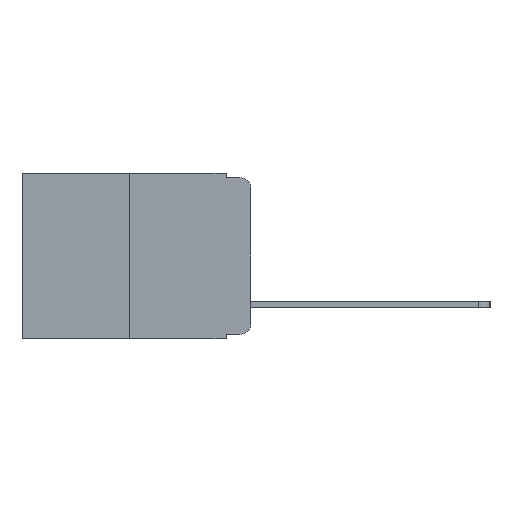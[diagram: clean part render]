
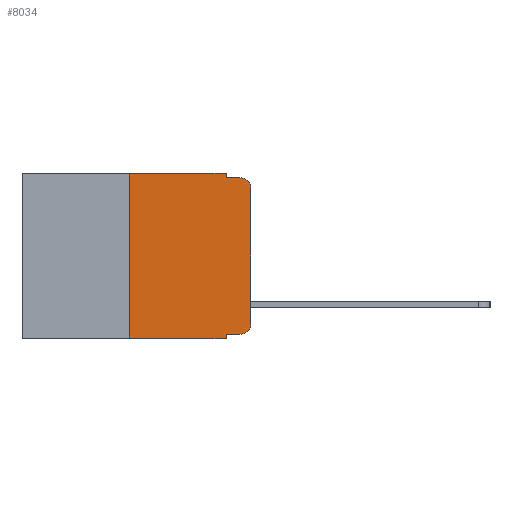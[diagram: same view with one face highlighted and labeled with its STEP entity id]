
A CAD part, left-side view. The second image highlights one B-rep face of the part: STEP entity #8034.
In plain terms, the highlighted planar face has unit normal (-1, 0, 0).
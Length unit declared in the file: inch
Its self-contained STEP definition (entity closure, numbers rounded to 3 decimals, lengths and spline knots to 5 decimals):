
#233 = LINE ( 'NONE', #6415, #13390 ) ;
#285 = VERTEX_POINT ( 'NONE', #4987 ) ;
#350 = ORIENTED_EDGE ( 'NONE', *, *, #11407, .F. ) ;
#664 = DIRECTION ( 'NONE',  ( 0., 0., -1. ) ) ;
#680 = DIRECTION ( 'NONE',  ( -1., 0., 0. ) ) ;
#689 = CARTESIAN_POINT ( 'NONE',  ( 0., 0.02, -0.313 ) ) ;
#702 = EDGE_CURVE ( 'NONE', #12066, #1483, #233, .T. ) ;
#890 = VECTOR ( 'NONE', #3801, 39.37008 ) ;
#897 = ORIENTED_EDGE ( 'NONE', *, *, #6186, .F. ) ;
#1015 = VECTOR ( 'NONE', #14543, 39.37008 ) ;
#1457 = LINE ( 'NONE', #11058, #1015 ) ;
#1483 = VERTEX_POINT ( 'NONE', #4992 ) ;
#1538 = ORIENTED_EDGE ( 'NONE', *, *, #5191, .T. ) ;
#1742 = ORIENTED_EDGE ( 'NONE', *, *, #8644, .F. ) ;
#2060 = EDGE_LOOP ( 'NONE', ( #12922, #13259, #15143, #15602, #350, #897, #1538, #1742, #2534, #3195 ) ) ;
#2399 = CARTESIAN_POINT ( 'NONE',  ( 0., 0.02, -0.01 ) ) ;
#2534 = ORIENTED_EDGE ( 'NONE', *, *, #10293, .T. ) ;
#2686 = VECTOR ( 'NONE', #12925, 39.37008 ) ;
#2846 = CARTESIAN_POINT ( 'NONE',  ( 0., 0.473, -0.343 ) ) ;
#3195 = ORIENTED_EDGE ( 'NONE', *, *, #10552, .T. ) ;
#3288 = LINE ( 'NONE', #2846, #10004 ) ;
#3662 = CARTESIAN_POINT ( 'NONE',  ( 0., 0.051, 0. ) ) ;
#3663 = DIRECTION ( 'NONE',  ( 0., 0., -1. ) ) ;
#3773 = AXIS2_PLACEMENT_3D ( 'NONE', #8592, #8574, #8566 ) ;
#3784 = VERTEX_POINT ( 'NONE', #5127 ) ;
#3801 = DIRECTION ( 'NONE',  ( 0., -1., 0. ) ) ;
#3824 = CARTESIAN_POINT ( 'NONE',  ( 0., 0.051, -0.333 ) ) ;
#4012 = VERTEX_POINT ( 'NONE', #7873 ) ;
#4554 = VECTOR ( 'NONE', #7910, 39.37008 ) ;
#4987 = CARTESIAN_POINT ( 'NONE',  ( 0., 0.02, -0.333 ) ) ;
#4992 = CARTESIAN_POINT ( 'NONE',  ( 0., 0.051, -0.01 ) ) ;
#5127 = CARTESIAN_POINT ( 'NONE',  ( 0., 0.25, -0.343 ) ) ;
#5191 = EDGE_CURVE ( 'NONE', #3784, #6270, #3288, .T. ) ;
#5583 = VERTEX_POINT ( 'NONE', #6214 ) ;
#5787 = CIRCLE ( 'NONE', #14899, 0.02 ) ;
#6186 = EDGE_CURVE ( 'NONE', #3784, #8235, #1457, .T. ) ;
#6214 = CARTESIAN_POINT ( 'NONE',  ( 0., 0., -0.313 ) ) ;
#6270 = VERTEX_POINT ( 'NONE', #13982 ) ;
#6306 = DIRECTION ( 'NONE',  ( 0., -1., 0. ) ) ;
#6415 = CARTESIAN_POINT ( 'NONE',  ( 0., 0.051, 0. ) ) ;
#6600 = CARTESIAN_POINT ( 'NONE',  ( 0., 0.051, -0.01 ) ) ;
#6687 = VECTOR ( 'NONE', #6306, 39.37008 ) ;
#7371 = CIRCLE ( 'NONE', #3773, 0.02 ) ;
#7519 = VERTEX_POINT ( 'NONE', #2399 ) ;
#7873 = CARTESIAN_POINT ( 'NONE',  ( 0., 0.051, -0.333 ) ) ;
#7910 = DIRECTION ( 'NONE',  ( 0., -1., 0. ) ) ;
#7965 = CARTESIAN_POINT ( 'NONE',  ( 0., 0.473, 0. ) ) ;
#7969 = LINE ( 'NONE', #14106, #13882 ) ;
#8034 = ADVANCED_FACE ( 'NONE', ( #8175 ), #15516, .F. ) ;
#8175 = FACE_OUTER_BOUND ( 'NONE', #2060, .T. ) ;
#8235 = VERTEX_POINT ( 'NONE', #10167 ) ;
#8566 = DIRECTION ( 'NONE',  ( 0., 0., -1. ) ) ;
#8574 = DIRECTION ( 'NONE',  ( -1., 0., 0. ) ) ;
#8592 = CARTESIAN_POINT ( 'NONE',  ( 0., 0.02, -0.03 ) ) ;
#8644 = EDGE_CURVE ( 'NONE', #4012, #6270, #7969, .T. ) ;
#8659 = VERTEX_POINT ( 'NONE', #13200 ) ;
#9055 = LINE ( 'NONE', #7965, #4554 ) ;
#9805 = EDGE_CURVE ( 'NONE', #8659, #7519, #7371, .T. ) ;
#10004 = VECTOR ( 'NONE', #11095, 39.37008 ) ;
#10167 = CARTESIAN_POINT ( 'NONE',  ( 0., 0.25, 0. ) ) ;
#10293 = EDGE_CURVE ( 'NONE', #4012, #285, #14494, .T. ) ;
#10336 = LINE ( 'NONE', #6600, #6687 ) ;
#10552 = EDGE_CURVE ( 'NONE', #285, #5583, #5787, .T. ) ;
#11058 = CARTESIAN_POINT ( 'NONE',  ( 0., 0.25, 0. ) ) ;
#11095 = DIRECTION ( 'NONE',  ( 0., -1., 0. ) ) ;
#11407 = EDGE_CURVE ( 'NONE', #8235, #12066, #9055, .T. ) ;
#11782 = CARTESIAN_POINT ( 'NONE',  ( 0., 0., 0. ) ) ;
#12066 = VERTEX_POINT ( 'NONE', #3662 ) ;
#12665 = LINE ( 'NONE', #11782, #2686 ) ;
#12922 = ORIENTED_EDGE ( 'NONE', *, *, #15735, .T. ) ;
#12925 = DIRECTION ( 'NONE',  ( 0., 0., 1. ) ) ;
#13200 = CARTESIAN_POINT ( 'NONE',  ( 0., 0., -0.03 ) ) ;
#13259 = ORIENTED_EDGE ( 'NONE', *, *, #9805, .T. ) ;
#13342 = EDGE_CURVE ( 'NONE', #1483, #7519, #10336, .T. ) ;
#13383 = AXIS2_PLACEMENT_3D ( 'NONE', #15455, #15409, #15298 ) ;
#13390 = VECTOR ( 'NONE', #3663, 39.37008 ) ;
#13542 = DIRECTION ( 'NONE',  ( 0., 0., -1. ) ) ;
#13882 = VECTOR ( 'NONE', #13542, 39.37008 ) ;
#13982 = CARTESIAN_POINT ( 'NONE',  ( 0., 0.051, -0.343 ) ) ;
#14106 = CARTESIAN_POINT ( 'NONE',  ( 0., 0.051, 0. ) ) ;
#14494 = LINE ( 'NONE', #3824, #890 ) ;
#14543 = DIRECTION ( 'NONE',  ( 0., 0., 1. ) ) ;
#14899 = AXIS2_PLACEMENT_3D ( 'NONE', #689, #680, #664 ) ;
#15143 = ORIENTED_EDGE ( 'NONE', *, *, #13342, .F. ) ;
#15298 = DIRECTION ( 'NONE',  ( 0., 0., -1. ) ) ;
#15409 = DIRECTION ( 'NONE',  ( 1., 0., 0. ) ) ;
#15455 = CARTESIAN_POINT ( 'NONE',  ( 0., 0.473, 0. ) ) ;
#15516 = PLANE ( 'NONE',  #13383 ) ;
#15602 = ORIENTED_EDGE ( 'NONE', *, *, #702, .F. ) ;
#15735 = EDGE_CURVE ( 'NONE', #5583, #8659, #12665, .T. ) ;
